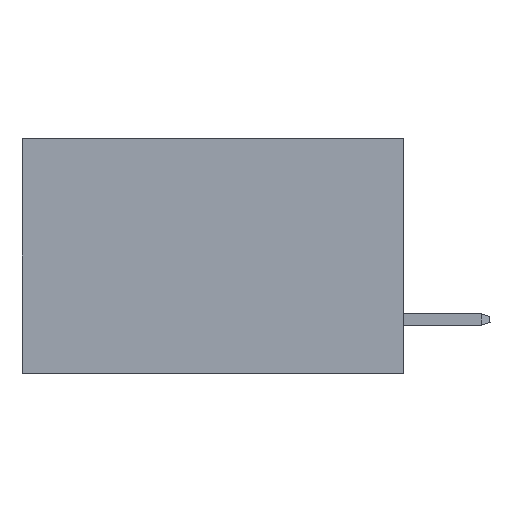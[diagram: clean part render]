
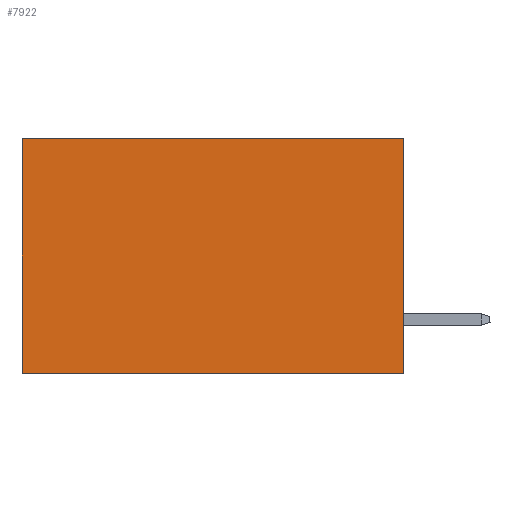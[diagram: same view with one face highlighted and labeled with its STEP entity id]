
A CAD part, left-side view. The second image highlights one B-rep face of the part: STEP entity #7922.
In plain terms, the highlighted planar face has unit normal (-1, 0, 0).
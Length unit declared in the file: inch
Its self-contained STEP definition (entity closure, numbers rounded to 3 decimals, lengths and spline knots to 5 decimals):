
#1143 = VECTOR ( 'NONE', #20235, 39.37008 ) ;
#3471 = CARTESIAN_POINT ( 'NONE',  ( 0.2875, 0.6, 0. ) ) ;
#3729 = LINE ( 'NONE', #14578, #3997 ) ;
#3997 = VECTOR ( 'NONE', #12509, 39.37008 ) ;
#4521 = EDGE_CURVE ( 'NONE', #25305, #15211, #14616, .T. ) ;
#4815 = EDGE_LOOP ( 'NONE', ( #24356, #8225, #11879, #20894 ) ) ;
#4858 = EDGE_CURVE ( 'NONE', #15211, #16455, #3729, .T. ) ;
#5450 = CARTESIAN_POINT ( 'NONE',  ( 0.2875, 0., 0. ) ) ;
#5564 = LINE ( 'NONE', #24316, #23426 ) ;
#7762 = CARTESIAN_POINT ( 'NONE',  ( 0.2875, 0., 0. ) ) ;
#7922 = ADVANCED_FACE ( 'NONE', ( #17067 ), #13497, .F. ) ;
#8225 = ORIENTED_EDGE ( 'NONE', *, *, #4858, .F. ) ;
#8715 = CARTESIAN_POINT ( 'NONE',  ( 0.2875, 0., 0. ) ) ;
#11879 = ORIENTED_EDGE ( 'NONE', *, *, #4521, .F. ) ;
#12509 = DIRECTION ( 'NONE',  ( 0., 1., 0. ) ) ;
#12985 = CARTESIAN_POINT ( 'NONE',  ( 0.2875, 0., -0.37 ) ) ;
#13166 = VERTEX_POINT ( 'NONE', #3471 ) ;
#13497 = PLANE ( 'NONE',  #21860 ) ;
#14578 = CARTESIAN_POINT ( 'NONE',  ( 0.2875, 0., -0.37 ) ) ;
#14616 = LINE ( 'NONE', #24597, #14922 ) ;
#14922 = VECTOR ( 'NONE', #22671, 39.37008 ) ;
#15032 = DIRECTION ( 'NONE',  ( 0., 0., -1. ) ) ;
#15211 = VERTEX_POINT ( 'NONE', #12985 ) ;
#15481 = EDGE_CURVE ( 'NONE', #13166, #16455, #5564, .T. ) ;
#16098 = DIRECTION ( 'NONE',  ( 0., 0., -1. ) ) ;
#16455 = VERTEX_POINT ( 'NONE', #26855 ) ;
#17067 = FACE_OUTER_BOUND ( 'NONE', #4815, .T. ) ;
#18380 = EDGE_CURVE ( 'NONE', #25305, #13166, #25982, .T. ) ;
#20235 = DIRECTION ( 'NONE',  ( 0., 1., 0. ) ) ;
#20894 = ORIENTED_EDGE ( 'NONE', *, *, #18380, .T. ) ;
#21860 = AXIS2_PLACEMENT_3D ( 'NONE', #8715, #25436, #15032 ) ;
#22671 = DIRECTION ( 'NONE',  ( 0., 0., -1. ) ) ;
#23426 = VECTOR ( 'NONE', #16098, 39.37008 ) ;
#24316 = CARTESIAN_POINT ( 'NONE',  ( 0.2875, 0.6, 0. ) ) ;
#24356 = ORIENTED_EDGE ( 'NONE', *, *, #15481, .T. ) ;
#24597 = CARTESIAN_POINT ( 'NONE',  ( 0.2875, 0., 0. ) ) ;
#25305 = VERTEX_POINT ( 'NONE', #7762 ) ;
#25436 = DIRECTION ( 'NONE',  ( 1., 0., 0. ) ) ;
#25982 = LINE ( 'NONE', #5450, #1143 ) ;
#26855 = CARTESIAN_POINT ( 'NONE',  ( 0.2875, 0.6, -0.37 ) ) ;
